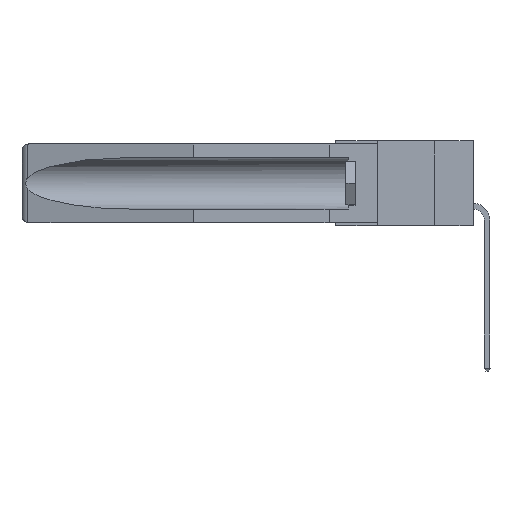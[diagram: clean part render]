
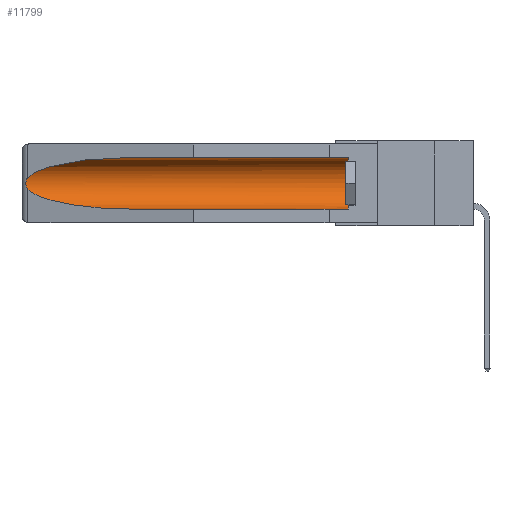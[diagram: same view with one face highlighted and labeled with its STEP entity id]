
A CAD part, left-side view. The second image highlights one B-rep face of the part: STEP entity #11799.
In plain terms, the highlighted cylindrical face has radius 2.857 mm (diameter 5.715 mm), a partial arc.
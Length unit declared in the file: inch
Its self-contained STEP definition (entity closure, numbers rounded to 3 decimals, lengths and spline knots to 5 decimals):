
#38 = ORIENTED_EDGE ( 'NONE', *, *, #3462, .T. ) ;
#487 = VERTEX_POINT ( 'NONE', #15862 ) ;
#875 = CARTESIAN_POINT ( 'NONE',  ( 0.26537, 1.52718, -0.19328 ) ) ;
#1081 =( BOUNDED_CURVE ( )  B_SPLINE_CURVE ( 3, ( #12160, #20784, #18985, #3588 ),
 .UNSPECIFIED., .F., .F. ) 
 B_SPLINE_CURVE_WITH_KNOTS ( ( 4, 4 ),
 ( 4.71239, 6.08839 ),
 .UNSPECIFIED. ) 
 CURVE ( )  GEOMETRIC_REPRESENTATION_ITEM ( )  RATIONAL_B_SPLINE_CURVE ( ( 1., 0.848, 0.848, 1. ) ) 
 REPRESENTATION_ITEM ( '' )  );
#1394 = EDGE_CURVE ( 'NONE', #487, #4232, #6692, .T. ) ;
#1832 = LINE ( 'NONE', #13972, #3737 ) ;
#2344 = EDGE_LOOP ( 'NONE', ( #4521, #18800, #12796, #19145, #38, #15777 ) ) ;
#2356 = VERTEX_POINT ( 'NONE', #16959 ) ;
#2949 = CIRCLE ( 'NONE', #7759, 0.1125 ) ;
#3344 = DIRECTION ( 'NONE',  ( 0., -1., 0. ) ) ;
#3462 = EDGE_CURVE ( 'NONE', #487, #12790, #2949, .T. ) ;
#3588 = CARTESIAN_POINT ( 'NONE',  ( 0.26537, 1.52718, -0.14972 ) ) ;
#3737 = VECTOR ( 'NONE', #19258, 39.37008 ) ;
#4232 = VERTEX_POINT ( 'NONE', #12317 ) ;
#4521 = ORIENTED_EDGE ( 'NONE', *, *, #15345, .T. ) ;
#4535 = EDGE_CURVE ( 'NONE', #12790, #13199, #1832, .T. ) ;
#4667 = VERTEX_POINT ( 'NONE', #20371 ) ;
#5122 = B_SPLINE_CURVE_WITH_KNOTS ( 'NONE', 3,
 ( #19298, #5791, #14737, #14515, #5993, #18006, #7687, #14461, #19724, #875 ),
 .UNSPECIFIED., .F., .F.,
 ( 4, 2, 2, 2, 4 ),
 ( 0., 0.00029, 0.00058, 0.00087, 0.00117 ),
 .UNSPECIFIED. ) ;
#5791 = CARTESIAN_POINT ( 'NONE',  ( 0.26597, 1.52961, -0.15275 ) ) ;
#5993 = CARTESIAN_POINT ( 'NONE',  ( 0.2675, 1.53308, -0.16763 ) ) ;
#6513 = CARTESIAN_POINT ( 'NONE',  ( 0.155, 0.126, -0.059 ) ) ;
#6642 = DIRECTION ( 'NONE',  ( 0., 1., 0. ) ) ;
#6692 = LINE ( 'NONE', #8860, #10953 ) ;
#7108 = CARTESIAN_POINT ( 'NONE',  ( 0.155, 1.07973, -0.059 ) ) ;
#7687 = CARTESIAN_POINT ( 'NONE',  ( 0.2673, 1.53269, -0.17917 ) ) ;
#7759 = AXIS2_PLACEMENT_3D ( 'NONE', #13574, #3344, #11689 ) ;
#8860 = CARTESIAN_POINT ( 'NONE',  ( 0.155, -0.30754, -0.284 ) ) ;
#9787 = CYLINDRICAL_SURFACE ( 'NONE', #11636, 0.1125 ) ;
#10873 = FACE_OUTER_BOUND ( 'NONE', #2344, .T. ) ;
#10953 = VECTOR ( 'NONE', #15737, 39.37008 ) ;
#11636 = AXIS2_PLACEMENT_3D ( 'NONE', #11782, #6642, #18755 ) ;
#11689 = DIRECTION ( 'NONE',  ( 0., 0., 1. ) ) ;
#11782 = CARTESIAN_POINT ( 'NONE',  ( 0.155, -0.30754, -0.1715 ) ) ;
#11799 = ADVANCED_FACE ( 'NONE', ( #10873 ), #9787, .F. ) ;
#12160 = CARTESIAN_POINT ( 'NONE',  ( 0.155, 1.07973, -0.059 ) ) ;
#12317 = CARTESIAN_POINT ( 'NONE',  ( 0.155, 1.07973, -0.284 ) ) ;
#12790 = VERTEX_POINT ( 'NONE', #6513 ) ;
#12796 = ORIENTED_EDGE ( 'NONE', *, *, #14077, .T. ) ;
#13199 = VERTEX_POINT ( 'NONE', #7108 ) ;
#13574 = CARTESIAN_POINT ( 'NONE',  ( 0.155, 0.126, -0.1715 ) ) ;
#13972 = CARTESIAN_POINT ( 'NONE',  ( 0.155, -0.30754, -0.059 ) ) ;
#14077 = EDGE_CURVE ( 'NONE', #4667, #4232, #21455, .T. ) ;
#14173 = CARTESIAN_POINT ( 'NONE',  ( 0.21114, 1.30732, -0.284 ) ) ;
#14461 = CARTESIAN_POINT ( 'NONE',  ( 0.26655, 1.53094, -0.18657 ) ) ;
#14515 = CARTESIAN_POINT ( 'NONE',  ( 0.2673, 1.5327, -0.16383 ) ) ;
#14737 = CARTESIAN_POINT ( 'NONE',  ( 0.26654, 1.53092, -0.15636 ) ) ;
#15345 = EDGE_CURVE ( 'NONE', #13199, #2356, #1081, .T. ) ;
#15737 = DIRECTION ( 'NONE',  ( 0., 1., 0. ) ) ;
#15777 = ORIENTED_EDGE ( 'NONE', *, *, #4535, .T. ) ;
#15844 = CARTESIAN_POINT ( 'NONE',  ( 0.25451, 1.48313, -0.24835 ) ) ;
#15862 = CARTESIAN_POINT ( 'NONE',  ( 0.155, 0.126, -0.284 ) ) ;
#16388 = EDGE_CURVE ( 'NONE', #2356, #4667, #5122, .T. ) ;
#16959 = CARTESIAN_POINT ( 'NONE',  ( 0.26537, 1.52718, -0.14972 ) ) ;
#17430 = CARTESIAN_POINT ( 'NONE',  ( 0.26537, 1.52718, -0.19328 ) ) ;
#17651 = CARTESIAN_POINT ( 'NONE',  ( 0.155, 1.07973, -0.284 ) ) ;
#18006 = CARTESIAN_POINT ( 'NONE',  ( 0.2675, 1.53308, -0.17534 ) ) ;
#18755 = DIRECTION ( 'NONE',  ( 0., 0., 1. ) ) ;
#18800 = ORIENTED_EDGE ( 'NONE', *, *, #16388, .T. ) ;
#18985 = CARTESIAN_POINT ( 'NONE',  ( 0.25451, 1.48313, -0.09465 ) ) ;
#19145 = ORIENTED_EDGE ( 'NONE', *, *, #1394, .F. ) ;
#19258 = DIRECTION ( 'NONE',  ( 0., 1., 0. ) ) ;
#19298 = CARTESIAN_POINT ( 'NONE',  ( 0.26537, 1.52718, -0.14972 ) ) ;
#19724 = CARTESIAN_POINT ( 'NONE',  ( 0.26597, 1.5296, -0.19026 ) ) ;
#20371 = CARTESIAN_POINT ( 'NONE',  ( 0.26537, 1.52718, -0.19328 ) ) ;
#20784 = CARTESIAN_POINT ( 'NONE',  ( 0.21114, 1.30732, -0.059 ) ) ;
#21455 =( BOUNDED_CURVE ( )  B_SPLINE_CURVE ( 3, ( #17430, #15844, #14173, #17651 ),
 .UNSPECIFIED., .F., .F. ) 
 B_SPLINE_CURVE_WITH_KNOTS ( ( 4, 4 ),
 ( 0.1948, 1.5708 ),
 .UNSPECIFIED. ) 
 CURVE ( )  GEOMETRIC_REPRESENTATION_ITEM ( )  RATIONAL_B_SPLINE_CURVE ( ( 1., 0.848, 0.848, 1. ) ) 
 REPRESENTATION_ITEM ( '' )  );
